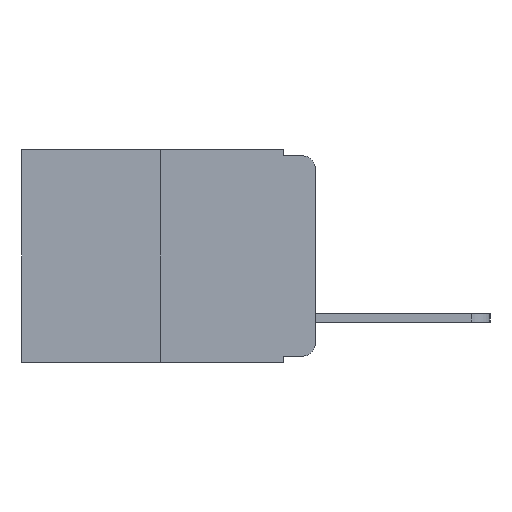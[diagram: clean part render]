
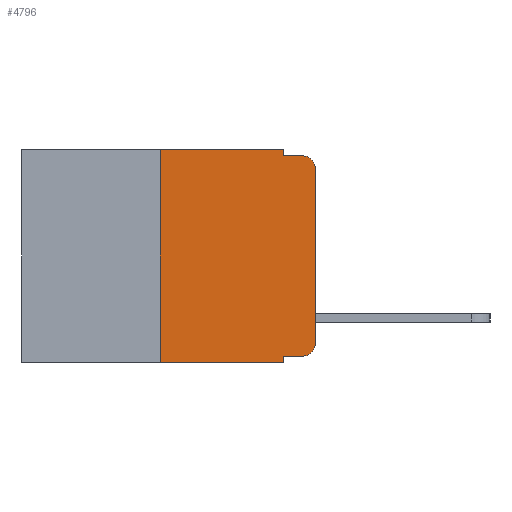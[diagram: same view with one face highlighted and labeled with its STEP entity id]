
A CAD part, left-side view. The second image highlights one B-rep face of the part: STEP entity #4796.
In plain terms, the highlighted planar face has unit normal (-1, 0, 0).
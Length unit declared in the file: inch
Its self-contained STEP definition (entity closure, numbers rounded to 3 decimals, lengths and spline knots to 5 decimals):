
#87 = VERTEX_POINT ( 'NONE', #6195 ) ;
#337 = ORIENTED_EDGE ( 'NONE', *, *, #16475, .F. ) ;
#545 = LINE ( 'NONE', #4716, #10798 ) ;
#585 = AXIS2_PLACEMENT_3D ( 'NONE', #876, #851, #834 ) ;
#588 = VERTEX_POINT ( 'NONE', #12651 ) ;
#834 = DIRECTION ( 'NONE',  ( 0., 0., -1. ) ) ;
#839 = DIRECTION ( 'NONE',  ( 0., 0., -1. ) ) ;
#851 = DIRECTION ( 'NONE',  ( -1., 0., 0. ) ) ;
#876 = CARTESIAN_POINT ( 'NONE',  ( 0., 0.02, -0.03 ) ) ;
#1211 = EDGE_CURVE ( 'NONE', #1645, #588, #13840, .T. ) ;
#1592 = EDGE_CURVE ( 'NONE', #87, #6097, #9851, .T. ) ;
#1645 = VERTEX_POINT ( 'NONE', #13723 ) ;
#1778 = CARTESIAN_POINT ( 'NONE',  ( 0., 0.051, 0. ) ) ;
#2029 = EDGE_CURVE ( 'NONE', #15487, #6097, #3677, .T. ) ;
#3279 = VECTOR ( 'NONE', #5031, 39.37008 ) ;
#3444 = CARTESIAN_POINT ( 'NONE',  ( 0., 0.051, 0. ) ) ;
#3677 = LINE ( 'NONE', #14401, #3279 ) ;
#3917 = ORIENTED_EDGE ( 'NONE', *, *, #2029, .F. ) ;
#3967 = LINE ( 'NONE', #10404, #7156 ) ;
#4469 = EDGE_CURVE ( 'NONE', #4750, #10539, #13762, .T. ) ;
#4582 = ORIENTED_EDGE ( 'NONE', *, *, #15010, .F. ) ;
#4716 = CARTESIAN_POINT ( 'NONE',  ( 0., 0.25, 0. ) ) ;
#4750 = VERTEX_POINT ( 'NONE', #1778 ) ;
#4788 = CARTESIAN_POINT ( 'NONE',  ( 0., 0.473, 0. ) ) ;
#4796 = ADVANCED_FACE ( 'NONE', ( #8851 ), #11874, .F. ) ;
#5031 = DIRECTION ( 'NONE',  ( 0., 0., -1. ) ) ;
#5267 = DIRECTION ( 'NONE',  ( 0., 0., 1. ) ) ;
#5457 = EDGE_CURVE ( 'NONE', #12766, #16199, #13194, .T. ) ;
#5824 = CARTESIAN_POINT ( 'NONE',  ( 0., 0.051, -0.333 ) ) ;
#5867 = DIRECTION ( 'NONE',  ( 0., -1., 0. ) ) ;
#5991 = AXIS2_PLACEMENT_3D ( 'NONE', #14605, #11597, #839 ) ;
#6049 = LINE ( 'NONE', #4788, #16308 ) ;
#6097 = VERTEX_POINT ( 'NONE', #13137 ) ;
#6195 = CARTESIAN_POINT ( 'NONE',  ( 0., 0.25, -0.343 ) ) ;
#6897 = ORIENTED_EDGE ( 'NONE', *, *, #1211, .T. ) ;
#6899 = CARTESIAN_POINT ( 'NONE',  ( 0., 0.25, 0. ) ) ;
#6986 = LINE ( 'NONE', #5824, #16362 ) ;
#7156 = VECTOR ( 'NONE', #5267, 39.37008 ) ;
#7317 = DIRECTION ( 'NONE',  ( 0., -1., 0. ) ) ;
#7472 = DIRECTION ( 'NONE',  ( 0., 0., -1. ) ) ;
#7479 = DIRECTION ( 'NONE',  ( -1., 0., 0. ) ) ;
#7565 = CARTESIAN_POINT ( 'NONE',  ( 0., 0.02, -0.313 ) ) ;
#8068 = EDGE_CURVE ( 'NONE', #10539, #588, #12970, .T. ) ;
#8514 = EDGE_CURVE ( 'NONE', #16199, #1645, #3967, .T. ) ;
#8570 = CARTESIAN_POINT ( 'NONE',  ( 0., 0.051, -0.01 ) ) ;
#8851 = FACE_OUTER_BOUND ( 'NONE', #11550, .T. ) ;
#9109 = CARTESIAN_POINT ( 'NONE',  ( 0., 0.02, -0.333 ) ) ;
#9468 = VECTOR ( 'NONE', #7317, 39.37008 ) ;
#9851 = LINE ( 'NONE', #10130, #9468 ) ;
#9857 = ORIENTED_EDGE ( 'NONE', *, *, #5457, .T. ) ;
#10130 = CARTESIAN_POINT ( 'NONE',  ( 0., 0.473, -0.343 ) ) ;
#10213 = ORIENTED_EDGE ( 'NONE', *, *, #8514, .T. ) ;
#10404 = CARTESIAN_POINT ( 'NONE',  ( 0., 0., 0. ) ) ;
#10539 = VERTEX_POINT ( 'NONE', #8570 ) ;
#10569 = VECTOR ( 'NONE', #15995, 39.37008 ) ;
#10626 = ORIENTED_EDGE ( 'NONE', *, *, #4469, .F. ) ;
#10798 = VECTOR ( 'NONE', #16007, 39.37008 ) ;
#11009 = DIRECTION ( 'NONE',  ( 0., -1., 0. ) ) ;
#11550 = EDGE_LOOP ( 'NONE', ( #10213, #6897, #13820, #10626, #4582, #337, #14971, #3917, #15920, #9857 ) ) ;
#11597 = DIRECTION ( 'NONE',  ( 1., 0., 0. ) ) ;
#11771 = VERTEX_POINT ( 'NONE', #6899 ) ;
#11864 = CARTESIAN_POINT ( 'NONE',  ( 0., 0., -0.313 ) ) ;
#11874 = PLANE ( 'NONE',  #5991 ) ;
#12403 = DIRECTION ( 'NONE',  ( 0., -1., 0. ) ) ;
#12651 = CARTESIAN_POINT ( 'NONE',  ( 0., 0.02, -0.01 ) ) ;
#12766 = VERTEX_POINT ( 'NONE', #9109 ) ;
#12970 = LINE ( 'NONE', #15794, #16160 ) ;
#12989 = CARTESIAN_POINT ( 'NONE',  ( 0., 0.051, -0.333 ) ) ;
#13062 = EDGE_CURVE ( 'NONE', #15487, #12766, #6986, .T. ) ;
#13137 = CARTESIAN_POINT ( 'NONE',  ( 0., 0.051, -0.343 ) ) ;
#13194 = CIRCLE ( 'NONE', #15067, 0.02 ) ;
#13723 = CARTESIAN_POINT ( 'NONE',  ( 0., 0., -0.03 ) ) ;
#13762 = LINE ( 'NONE', #3444, #10569 ) ;
#13820 = ORIENTED_EDGE ( 'NONE', *, *, #8068, .F. ) ;
#13840 = CIRCLE ( 'NONE', #585, 0.02 ) ;
#14401 = CARTESIAN_POINT ( 'NONE',  ( 0., 0.051, 0. ) ) ;
#14605 = CARTESIAN_POINT ( 'NONE',  ( 0., 0.473, 0. ) ) ;
#14971 = ORIENTED_EDGE ( 'NONE', *, *, #1592, .T. ) ;
#15010 = EDGE_CURVE ( 'NONE', #11771, #4750, #6049, .T. ) ;
#15067 = AXIS2_PLACEMENT_3D ( 'NONE', #7565, #7479, #7472 ) ;
#15487 = VERTEX_POINT ( 'NONE', #12989 ) ;
#15794 = CARTESIAN_POINT ( 'NONE',  ( 0., 0.051, -0.01 ) ) ;
#15920 = ORIENTED_EDGE ( 'NONE', *, *, #13062, .T. ) ;
#15995 = DIRECTION ( 'NONE',  ( 0., 0., -1. ) ) ;
#16007 = DIRECTION ( 'NONE',  ( 0., 0., 1. ) ) ;
#16160 = VECTOR ( 'NONE', #5867, 39.37008 ) ;
#16199 = VERTEX_POINT ( 'NONE', #11864 ) ;
#16308 = VECTOR ( 'NONE', #12403, 39.37008 ) ;
#16362 = VECTOR ( 'NONE', #11009, 39.37008 ) ;
#16475 = EDGE_CURVE ( 'NONE', #87, #11771, #545, .T. ) ;
